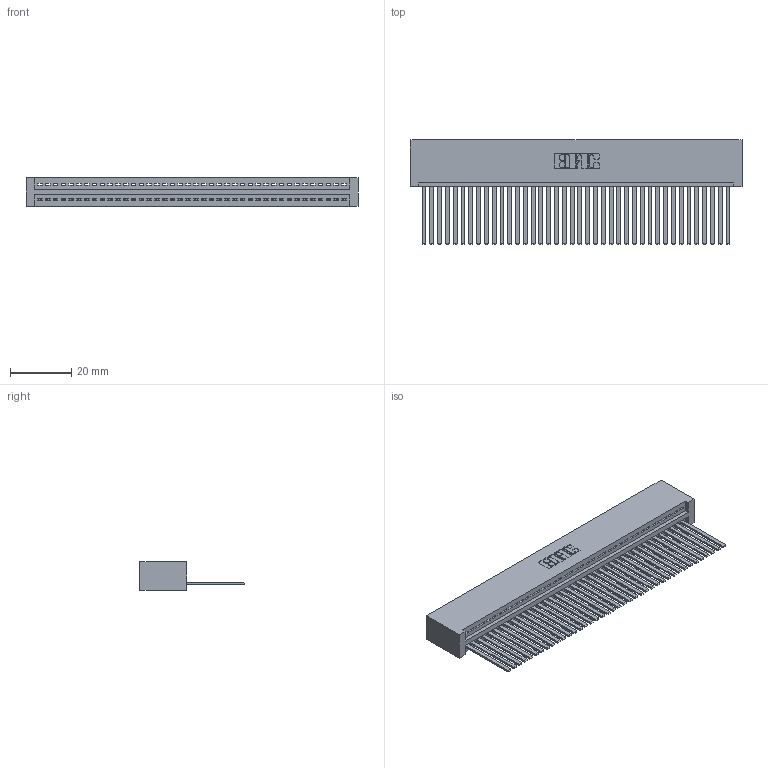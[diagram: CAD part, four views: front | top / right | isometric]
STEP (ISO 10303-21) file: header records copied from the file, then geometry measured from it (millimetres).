
FILE_DESCRIPTION (( 'STEP AP203' ), '1' );
FILE_NAME ('395-040-544-101.STEP', '2019-10-22T05:49:26', ( '' ), ( '' ), 'SwSTEP 2.0', 'SolidWorks 2016', '' );
FILE_SCHEMA (( 'CONFIG_CONTROL_DESIGN' ));
Length unit declared in the file: inch
Products named in the file (3): 345 Part_No Mounting Lugs; 345-292-001_345-293-144; 395-040-544-101
Assembly tree (41 placements, depth 2):
  395-040-544-101
    345 Part_No Mounting Lugs
    345-292-001_345-293-144  x40
Bounding box: 108.2 x 33.96 x 9.4 mm (x, y, z)
Volume: 11308.6 mm3; surface area: 16581.7 mm2
Topology: 41 solids, 41 shells, 2198 faces, 6637 edges, 4370 vertices
Faces by surface type: plane 1516, cylinder 682
Entity records: 29913 total; most frequent: CARTESIAN_POINT 5188, ORIENTED_EDGE 5162, DIRECTION 4525, EDGE_CURVE 2581, VECTOR 2301, LINE 2301, VERTEX_POINT 1718, AXIS2_PLACEMENT_3D 1112
